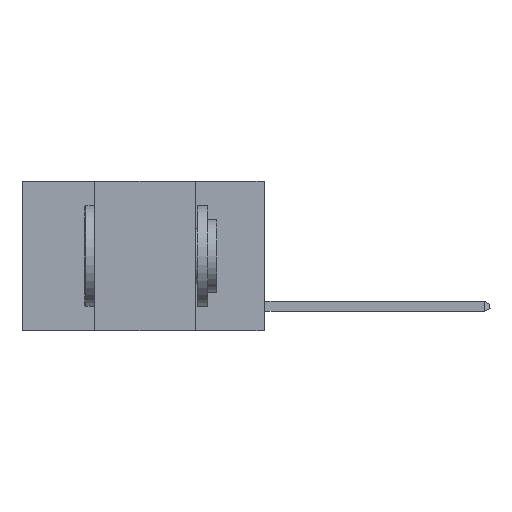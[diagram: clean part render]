
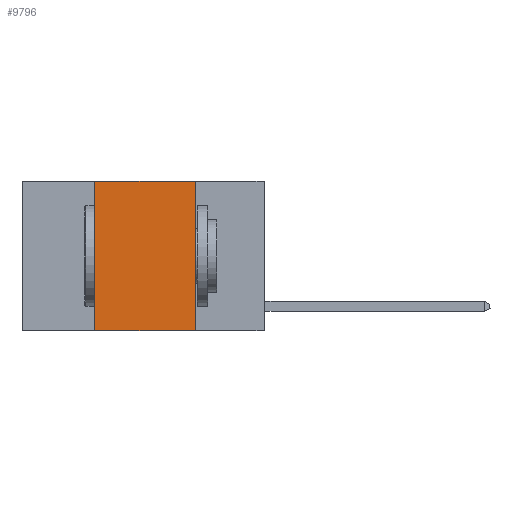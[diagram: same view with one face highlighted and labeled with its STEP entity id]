
A CAD part, left-side view. The second image highlights one B-rep face of the part: STEP entity #9796.
In plain terms, the highlighted planar face has unit normal (-1, 0, 0).
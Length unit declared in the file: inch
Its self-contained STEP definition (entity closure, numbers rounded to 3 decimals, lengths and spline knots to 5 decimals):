
#449 = CARTESIAN_POINT ( 'NONE',  ( 0., 0.6, 0. ) ) ;
#593 = EDGE_CURVE ( 'NONE', #2154, #4750, #9632, .T. ) ;
#610 = LINE ( 'NONE', #5273, #9982 ) ;
#1130 = EDGE_CURVE ( 'NONE', #4750, #9657, #610, .T. ) ;
#1452 = VECTOR ( 'NONE', #6363, 39.37008 ) ;
#1757 = ORIENTED_EDGE ( 'NONE', *, *, #8939, .F. ) ;
#1898 = DIRECTION ( 'NONE',  ( 0., 0., -1. ) ) ;
#2010 = DIRECTION ( 'NONE',  ( 1., 0., 0. ) ) ;
#2154 = VERTEX_POINT ( 'NONE', #8014 ) ;
#2814 = ORIENTED_EDGE ( 'NONE', *, *, #2962, .T. ) ;
#2962 = EDGE_CURVE ( 'NONE', #2154, #6569, #8691, .T. ) ;
#3176 = CARTESIAN_POINT ( 'NONE',  ( 0., 0.17, 0. ) ) ;
#4728 = CARTESIAN_POINT ( 'NONE',  ( 0., 0.17, -0.37 ) ) ;
#4750 = VERTEX_POINT ( 'NONE', #10014 ) ;
#5273 = CARTESIAN_POINT ( 'NONE',  ( 0., 0.6, 0. ) ) ;
#5331 = DIRECTION ( 'NONE',  ( 0., 0., 1. ) ) ;
#6210 = EDGE_LOOP ( 'NONE', ( #1757, #8136, #9030, #2814 ) ) ;
#6363 = DIRECTION ( 'NONE',  ( 0., -1., 0. ) ) ;
#6569 = VERTEX_POINT ( 'NONE', #4728 ) ;
#7329 = PLANE ( 'NONE',  #9140 ) ;
#7567 = FACE_OUTER_BOUND ( 'NONE', #6210, .T. ) ;
#8014 = CARTESIAN_POINT ( 'NONE',  ( 0., 0.42, -0.37 ) ) ;
#8063 = CARTESIAN_POINT ( 'NONE',  ( 0., 0.42, 0. ) ) ;
#8136 = ORIENTED_EDGE ( 'NONE', *, *, #1130, .F. ) ;
#8290 = VECTOR ( 'NONE', #1898, 39.37008 ) ;
#8441 = DIRECTION ( 'NONE',  ( 0., -1., 0. ) ) ;
#8527 = CARTESIAN_POINT ( 'NONE',  ( 0., 0.6, -0.37 ) ) ;
#8558 = VECTOR ( 'NONE', #5331, 39.37008 ) ;
#8691 = LINE ( 'NONE', #8527, #1452 ) ;
#8939 = EDGE_CURVE ( 'NONE', #9657, #6569, #9896, .T. ) ;
#9000 = CARTESIAN_POINT ( 'NONE',  ( 0., 0.17, 0. ) ) ;
#9030 = ORIENTED_EDGE ( 'NONE', *, *, #593, .F. ) ;
#9140 = AXIS2_PLACEMENT_3D ( 'NONE', #449, #2010, #9912 ) ;
#9632 = LINE ( 'NONE', #8063, #8558 ) ;
#9657 = VERTEX_POINT ( 'NONE', #3176 ) ;
#9796 = ADVANCED_FACE ( 'NONE', ( #7567 ), #7329, .F. ) ;
#9896 = LINE ( 'NONE', #9000, #8290 ) ;
#9912 = DIRECTION ( 'NONE',  ( 0., 0., -1. ) ) ;
#9982 = VECTOR ( 'NONE', #8441, 39.37008 ) ;
#10014 = CARTESIAN_POINT ( 'NONE',  ( 0., 0.42, 0. ) ) ;
